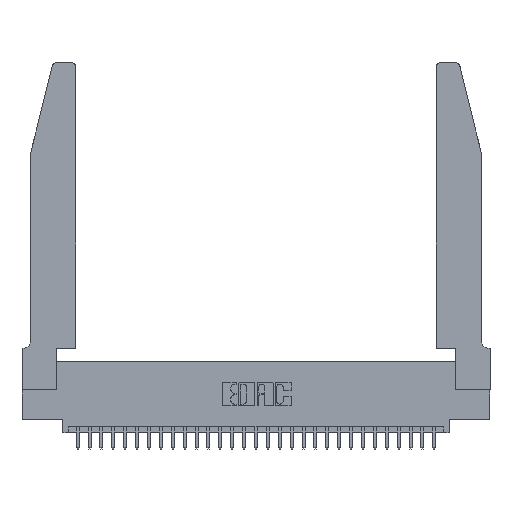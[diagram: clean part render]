
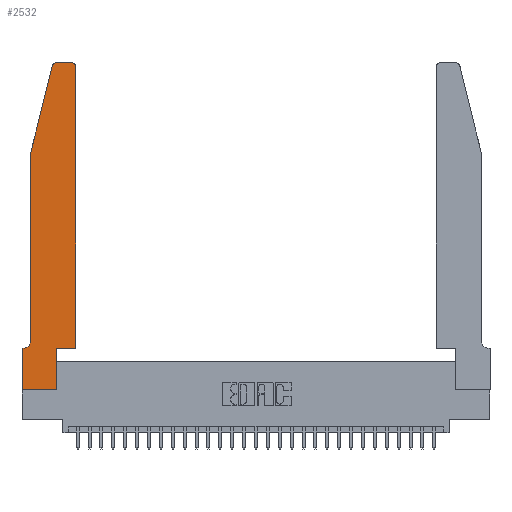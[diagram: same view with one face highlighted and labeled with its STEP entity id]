
A CAD part, top view. The second image highlights one B-rep face of the part: STEP entity #2532.
In plain terms, the highlighted planar face has unit normal (0, 0, 1).
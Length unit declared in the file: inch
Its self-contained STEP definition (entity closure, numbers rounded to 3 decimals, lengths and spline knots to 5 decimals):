
#245 = DIRECTION ( 'NONE',  ( -1., 0., 0. ) ) ;
#259 = EDGE_CURVE ( 'NONE', #17369, #773, #10240, .T. ) ;
#514 = DIRECTION ( 'NONE',  ( 1., 0., 0. ) ) ;
#729 = CARTESIAN_POINT ( 'NONE',  ( 0.0755, 2., 0.37 ) ) ;
#773 = VERTEX_POINT ( 'NONE', #18040 ) ;
#1383 = CARTESIAN_POINT ( 'NONE',  ( 0.0755, 0.42, 0.37 ) ) ;
#1421 = CARTESIAN_POINT ( 'NONE',  ( 0.284, 2.72, 0.37 ) ) ;
#1436 = VECTOR ( 'NONE', #22710, 39.37008 ) ;
#1705 = CARTESIAN_POINT ( 'NONE',  ( 0., 0.35, 0.37 ) ) ;
#1815 = LINE ( 'NONE', #15540, #1436 ) ;
#2532 = ADVANCED_FACE ( 'NONE', ( #19411 ), #20834, .T. ) ;
#2573 = VERTEX_POINT ( 'NONE', #30022 ) ;
#2708 = AXIS2_PLACEMENT_3D ( 'NONE', #1421, #20127, #5940 ) ;
#2875 = VECTOR ( 'NONE', #245, 39.37008 ) ;
#3097 = EDGE_CURVE ( 'NONE', #3935, #24314, #14171, .T. ) ;
#3699 = CARTESIAN_POINT ( 'NONE',  ( 0.0755, 2., 0.37 ) ) ;
#3935 = VERTEX_POINT ( 'NONE', #1383 ) ;
#4998 = CARTESIAN_POINT ( 'NONE',  ( 0., 0., 0.37 ) ) ;
#5167 = CARTESIAN_POINT ( 'NONE',  ( 0.2865, 0., 0.37 ) ) ;
#5567 = EDGE_CURVE ( 'NONE', #12066, #16044, #14748, .T. ) ;
#5940 = DIRECTION ( 'NONE',  ( 1., 0., 0. ) ) ;
#6623 = EDGE_CURVE ( 'NONE', #24928, #3935, #8722, .T. ) ;
#6813 = CARTESIAN_POINT ( 'NONE',  ( 0., 0.35, 0.37 ) ) ;
#7039 = DIRECTION ( 'NONE',  ( 0., 0., -1. ) ) ;
#7185 = VERTEX_POINT ( 'NONE', #6813 ) ;
#7226 = CIRCLE ( 'NONE', #2708, 0.03 ) ;
#7479 = LINE ( 'NONE', #12415, #20935 ) ;
#7561 = CARTESIAN_POINT ( 'NONE',  ( 0.4205, 2.72, 0.37 ) ) ;
#8145 = DIRECTION ( 'NONE',  ( 0., 1., 0. ) ) ;
#8245 = CARTESIAN_POINT ( 'NONE',  ( 0.0055, 0.35, 0.37 ) ) ;
#8657 = VERTEX_POINT ( 'NONE', #5167 ) ;
#8722 = LINE ( 'NONE', #729, #12078 ) ;
#8827 = ORIENTED_EDGE ( 'NONE', *, *, #26625, .T. ) ;
#9036 = ORIENTED_EDGE ( 'NONE', *, *, #5567, .T. ) ;
#9505 = LINE ( 'NONE', #27044, #25499 ) ;
#9684 = DIRECTION ( 'NONE',  ( -0.239, -0.971, 0. ) ) ;
#10240 = LINE ( 'NONE', #21625, #19949 ) ;
#10248 = LINE ( 'NONE', #11593, #22935 ) ;
#11345 = CARTESIAN_POINT ( 'NONE',  ( 0., 0., 0.37 ) ) ;
#11593 = CARTESIAN_POINT ( 'NONE',  ( 0.0755, 2., 0.37 ) ) ;
#11882 = ORIENTED_EDGE ( 'NONE', *, *, #259, .T. ) ;
#12042 = CARTESIAN_POINT ( 'NONE',  ( 0.0055, 0.42, 0.37 ) ) ;
#12066 = VERTEX_POINT ( 'NONE', #13369 ) ;
#12078 = VECTOR ( 'NONE', #22152, 39.37008 ) ;
#12343 = ORIENTED_EDGE ( 'NONE', *, *, #30562, .T. ) ;
#12362 = DIRECTION ( 'NONE',  ( 0., 0., 1. ) ) ;
#12415 = CARTESIAN_POINT ( 'NONE',  ( 0.4505, 0.35, 0.37 ) ) ;
#12470 = EDGE_CURVE ( 'NONE', #16730, #8657, #1815, .T. ) ;
#13369 = CARTESIAN_POINT ( 'NONE',  ( 0.4205, 2.75, 0.37 ) ) ;
#13691 = EDGE_CURVE ( 'NONE', #7185, #16730, #27313, .T. ) ;
#13748 = DIRECTION ( 'NONE',  ( 1., 0., 0. ) ) ;
#14054 = ORIENTED_EDGE ( 'NONE', *, *, #3097, .T. ) ;
#14171 = CIRCLE ( 'NONE', #14947, 0.07 ) ;
#14335 = EDGE_LOOP ( 'NONE', ( #9036, #12343, #14973, #20287, #14054, #16751, #19974, #19681, #19458, #23441, #11882, #8827 ) ) ;
#14748 = LINE ( 'NONE', #17452, #2875 ) ;
#14947 = AXIS2_PLACEMENT_3D ( 'NONE', #12042, #7039, #21427 ) ;
#14973 = ORIENTED_EDGE ( 'NONE', *, *, #18070, .T. ) ;
#15532 = EDGE_CURVE ( 'NONE', #30085, #17369, #7479, .T. ) ;
#15540 = CARTESIAN_POINT ( 'NONE',  ( 0., 0., 0.37 ) ) ;
#15965 = CIRCLE ( 'NONE', #18098, 0.03 ) ;
#16044 = VERTEX_POINT ( 'NONE', #18545 ) ;
#16730 = VERTEX_POINT ( 'NONE', #4998 ) ;
#16751 = ORIENTED_EDGE ( 'NONE', *, *, #26087, .T. ) ;
#16919 = DIRECTION ( 'NONE',  ( 1., 0., 0. ) ) ;
#17059 = DIRECTION ( 'NONE',  ( 0., 1., 0. ) ) ;
#17164 = AXIS2_PLACEMENT_3D ( 'NONE', #1705, #20733, #13748 ) ;
#17369 = VERTEX_POINT ( 'NONE', #30598 ) ;
#17452 = CARTESIAN_POINT ( 'NONE',  ( 0.2605, 2.75, 0.37 ) ) ;
#18040 = CARTESIAN_POINT ( 'NONE',  ( 0.4505, 2.72, 0.37 ) ) ;
#18070 = EDGE_CURVE ( 'NONE', #2573, #24928, #10248, .T. ) ;
#18098 = AXIS2_PLACEMENT_3D ( 'NONE', #7561, #12362, #514 ) ;
#18440 = DIRECTION ( 'NONE',  ( 0., -1., 0. ) ) ;
#18545 = CARTESIAN_POINT ( 'NONE',  ( 0.284, 2.75, 0.37 ) ) ;
#19411 = FACE_OUTER_BOUND ( 'NONE', #14335, .T. ) ;
#19458 = ORIENTED_EDGE ( 'NONE', *, *, #29775, .T. ) ;
#19681 = ORIENTED_EDGE ( 'NONE', *, *, #12470, .T. ) ;
#19949 = VECTOR ( 'NONE', #17059, 39.37008 ) ;
#19974 = ORIENTED_EDGE ( 'NONE', *, *, #13691, .T. ) ;
#20127 = DIRECTION ( 'NONE',  ( 0., 0., 1. ) ) ;
#20287 = ORIENTED_EDGE ( 'NONE', *, *, #6623, .T. ) ;
#20733 = DIRECTION ( 'NONE',  ( 0., 0., 1. ) ) ;
#20834 = PLANE ( 'NONE',  #17164 ) ;
#20935 = VECTOR ( 'NONE', #16919, 39.37008 ) ;
#21210 = VECTOR ( 'NONE', #29206, 39.37008 ) ;
#21427 = DIRECTION ( 'NONE',  ( -1., 0., 0. ) ) ;
#21625 = CARTESIAN_POINT ( 'NONE',  ( 0.4505, 0.35, 0.37 ) ) ;
#22152 = DIRECTION ( 'NONE',  ( 0., -1., 0. ) ) ;
#22329 = LINE ( 'NONE', #27113, #21210 ) ;
#22710 = DIRECTION ( 'NONE',  ( 1., 0., 0. ) ) ;
#22935 = VECTOR ( 'NONE', #9684, 39.37008 ) ;
#23441 = ORIENTED_EDGE ( 'NONE', *, *, #15532, .T. ) ;
#24314 = VERTEX_POINT ( 'NONE', #8245 ) ;
#24928 = VERTEX_POINT ( 'NONE', #3699 ) ;
#25499 = VECTOR ( 'NONE', #8145, 39.37008 ) ;
#25830 = VECTOR ( 'NONE', #18440, 39.37008 ) ;
#26087 = EDGE_CURVE ( 'NONE', #24314, #7185, #22329, .T. ) ;
#26625 = EDGE_CURVE ( 'NONE', #773, #12066, #15965, .T. ) ;
#27044 = CARTESIAN_POINT ( 'NONE',  ( 0.2865, 0.35, 0.37 ) ) ;
#27113 = CARTESIAN_POINT ( 'NONE',  ( 0.0755, 0.35, 0.37 ) ) ;
#27313 = LINE ( 'NONE', #11345, #25830 ) ;
#29206 = DIRECTION ( 'NONE',  ( -1., 0., 0. ) ) ;
#29775 = EDGE_CURVE ( 'NONE', #8657, #30085, #9505, .T. ) ;
#30022 = CARTESIAN_POINT ( 'NONE',  ( 0.25487, 2.72718, 0.37 ) ) ;
#30085 = VERTEX_POINT ( 'NONE', #30569 ) ;
#30562 = EDGE_CURVE ( 'NONE', #16044, #2573, #7226, .T. ) ;
#30569 = CARTESIAN_POINT ( 'NONE',  ( 0.2865, 0.35, 0.37 ) ) ;
#30598 = CARTESIAN_POINT ( 'NONE',  ( 0.4505, 0.35, 0.37 ) ) ;
